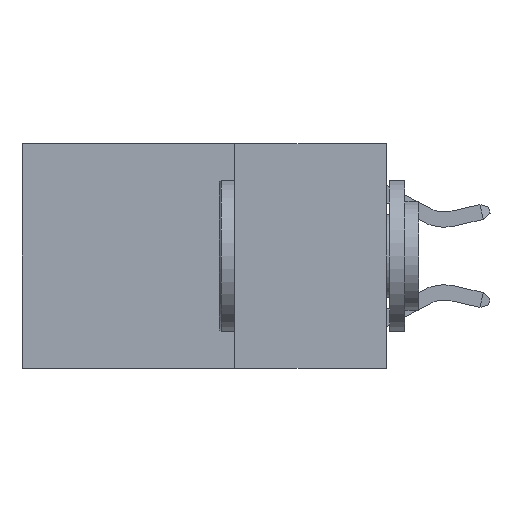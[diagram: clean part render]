
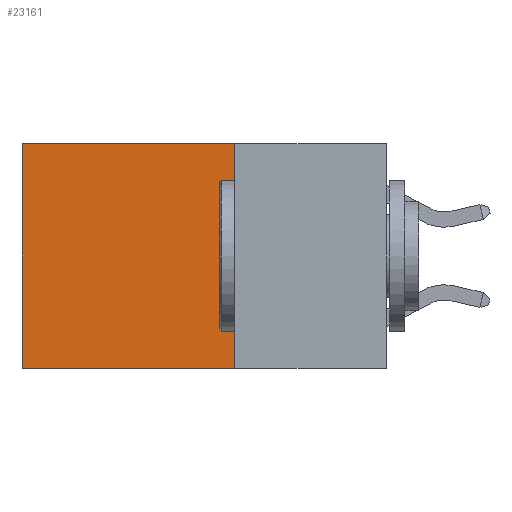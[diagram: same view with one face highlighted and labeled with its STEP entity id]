
A CAD part, left-side view. The second image highlights one B-rep face of the part: STEP entity #23161.
In plain terms, the highlighted planar face has unit normal (-1, 0, 0).
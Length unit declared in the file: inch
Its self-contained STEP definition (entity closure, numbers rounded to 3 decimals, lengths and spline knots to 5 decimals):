
#21 = EDGE_CURVE ( 'NONE', #13498, #11554, #18499, .T. ) ;
#27 = EDGE_CURVE ( 'NONE', #22202, #8937, #9002, .T. ) ;
#37 = AXIS2_PLACEMENT_3D ( 'NONE', #232, #22289, #16256 ) ;
#232 = CARTESIAN_POINT ( 'NONE',  ( 0.2625, 0.25, 0. ) ) ;
#702 = EDGE_CURVE ( 'NONE', #11554, #8937, #23542, .T. ) ;
#1314 = FACE_OUTER_BOUND ( 'NONE', #8977, .T. ) ;
#1375 = DIRECTION ( 'NONE',  ( 0., 1., 0. ) ) ;
#1459 = CARTESIAN_POINT ( 'NONE',  ( 0.2625, 0.25, -0.37 ) ) ;
#1655 = CARTESIAN_POINT ( 'NONE',  ( 0.2625, 0.25, 0. ) ) ;
#1835 = CARTESIAN_POINT ( 'NONE',  ( 0.2625, 0.25, -0.37 ) ) ;
#3264 = VECTOR ( 'NONE', #15237, 39.37008 ) ;
#4811 = DIRECTION ( 'NONE',  ( 0., 0., -1. ) ) ;
#7211 = CARTESIAN_POINT ( 'NONE',  ( 0.2625, 0.25, 0. ) ) ;
#8937 = VERTEX_POINT ( 'NONE', #16643 ) ;
#8977 = EDGE_LOOP ( 'NONE', ( #20100, #24419, #22125, #14947 ) ) ;
#9002 = LINE ( 'NONE', #9333, #3264 ) ;
#9333 = CARTESIAN_POINT ( 'NONE',  ( 0.2625, 0.6, 0. ) ) ;
#11554 = VERTEX_POINT ( 'NONE', #1835 ) ;
#13498 = VERTEX_POINT ( 'NONE', #1655 ) ;
#14947 = ORIENTED_EDGE ( 'NONE', *, *, #21979, .T. ) ;
#15237 = DIRECTION ( 'NONE',  ( 0., 0., -1. ) ) ;
#16256 = DIRECTION ( 'NONE',  ( 0., 0., -1. ) ) ;
#16616 = LINE ( 'NONE', #19237, #21360 ) ;
#16643 = CARTESIAN_POINT ( 'NONE',  ( 0.2625, 0.6, -0.37 ) ) ;
#18499 = LINE ( 'NONE', #7211, #19726 ) ;
#19023 = CARTESIAN_POINT ( 'NONE',  ( 0.2625, 0.6, 0. ) ) ;
#19237 = CARTESIAN_POINT ( 'NONE',  ( 0.2625, 0.25, 0. ) ) ;
#19726 = VECTOR ( 'NONE', #4811, 39.37008 ) ;
#19731 = DIRECTION ( 'NONE',  ( 0., 1., 0. ) ) ;
#20100 = ORIENTED_EDGE ( 'NONE', *, *, #27, .T. ) ;
#21360 = VECTOR ( 'NONE', #19731, 39.37008 ) ;
#21979 = EDGE_CURVE ( 'NONE', #13498, #22202, #16616, .T. ) ;
#22125 = ORIENTED_EDGE ( 'NONE', *, *, #21, .F. ) ;
#22202 = VERTEX_POINT ( 'NONE', #19023 ) ;
#22256 = VECTOR ( 'NONE', #1375, 39.37008 ) ;
#22289 = DIRECTION ( 'NONE',  ( 1., 0., 0. ) ) ;
#22568 = PLANE ( 'NONE',  #37 ) ;
#23161 = ADVANCED_FACE ( 'NONE', ( #1314 ), #22568, .F. ) ;
#23542 = LINE ( 'NONE', #1459, #22256 ) ;
#24419 = ORIENTED_EDGE ( 'NONE', *, *, #702, .F. ) ;
